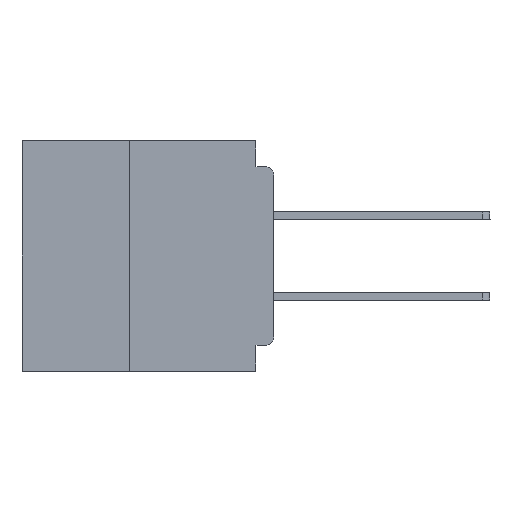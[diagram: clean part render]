
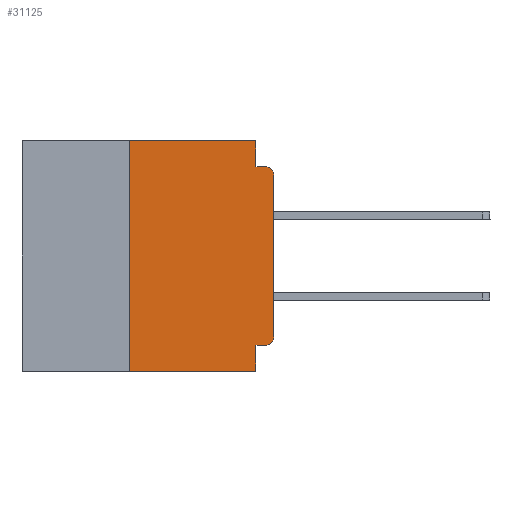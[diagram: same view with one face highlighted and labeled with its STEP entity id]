
A CAD part, left-side view. The second image highlights one B-rep face of the part: STEP entity #31125.
In plain terms, the highlighted planar face has unit normal (-1, 0, 0).
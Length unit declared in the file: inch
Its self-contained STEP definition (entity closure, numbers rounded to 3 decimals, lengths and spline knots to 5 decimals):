
#2431 = CARTESIAN_POINT ( 'NONE',  ( 0., 0.015, -0.34 ) ) ;
#4102 = PLANE ( 'NONE',  #14447 ) ;
#5259 = CARTESIAN_POINT ( 'NONE',  ( 0., 0.031, -0.045 ) ) ;
#5685 = CARTESIAN_POINT ( 'NONE',  ( 0., 0., -0.355 ) ) ;
#7285 = CARTESIAN_POINT ( 'NONE',  ( 0., 0., -0.045 ) ) ;
#7587 = DIRECTION ( 'NONE',  ( 0., 0., -1. ) ) ;
#7605 = ORIENTED_EDGE ( 'NONE', *, *, #59686, .F. ) ;
#8514 = VECTOR ( 'NONE', #66152, 39.37008 ) ;
#8557 = CARTESIAN_POINT ( 'NONE',  ( 0., 0., 0. ) ) ;
#10841 = AXIS2_PLACEMENT_3D ( 'NONE', #59793, #29209, #64865 ) ;
#10844 = DIRECTION ( 'NONE',  ( 0., 1., 0. ) ) ;
#11121 = VERTEX_POINT ( 'NONE', #42803 ) ;
#11649 = VECTOR ( 'NONE', #18840, 39.37008 ) ;
#12291 = AXIS2_PLACEMENT_3D ( 'NONE', #2431, #38357, #7587 ) ;
#12451 = DIRECTION ( 'NONE',  ( 0., -1., 0. ) ) ;
#13256 = VERTEX_POINT ( 'NONE', #27277 ) ;
#13714 = DIRECTION ( 'NONE',  ( 0., 0., 1. ) ) ;
#13742 = LINE ( 'NONE', #7285, #25807 ) ;
#14447 = AXIS2_PLACEMENT_3D ( 'NONE', #50246, #19533, #55405 ) ;
#15932 = ORIENTED_EDGE ( 'NONE', *, *, #49426, .T. ) ;
#17462 = VERTEX_POINT ( 'NONE', #36136 ) ;
#18364 = EDGE_CURVE ( 'NONE', #42436, #30151, #13742, .T. ) ;
#18504 = VECTOR ( 'NONE', #10844, 39.37008 ) ;
#18840 = DIRECTION ( 'NONE',  ( 0., 0., -1. ) ) ;
#18987 = VERTEX_POINT ( 'NONE', #60850 ) ;
#19533 = DIRECTION ( 'NONE',  ( 1., 0., 0. ) ) ;
#19624 = CARTESIAN_POINT ( 'NONE',  ( 0., 0.015, -0.355 ) ) ;
#20550 = EDGE_CURVE ( 'NONE', #44122, #23232, #44822, .T. ) ;
#21375 = CARTESIAN_POINT ( 'NONE',  ( 0., 0.031, -0.355 ) ) ;
#21750 = LINE ( 'NONE', #5685, #18504 ) ;
#23232 = VERTEX_POINT ( 'NONE', #45274 ) ;
#23278 = FACE_OUTER_BOUND ( 'NONE', #48159, .T. ) ;
#24277 = LINE ( 'NONE', #8557, #49921 ) ;
#24663 = CARTESIAN_POINT ( 'NONE',  ( 0., 0.437, -0.4 ) ) ;
#25420 = EDGE_CURVE ( 'NONE', #18987, #42436, #64444, .T. ) ;
#25807 = VECTOR ( 'NONE', #12451, 39.37008 ) ;
#27022 = ORIENTED_EDGE ( 'NONE', *, *, #25420, .F. ) ;
#27277 = CARTESIAN_POINT ( 'NONE',  ( 0., 0.25, -0.4 ) ) ;
#27496 = ORIENTED_EDGE ( 'NONE', *, *, #42465, .F. ) ;
#28491 = VECTOR ( 'NONE', #50415, 39.37008 ) ;
#28843 = LINE ( 'NONE', #61373, #42438 ) ;
#29209 = DIRECTION ( 'NONE',  ( -1., 0., 0. ) ) ;
#30151 = VERTEX_POINT ( 'NONE', #47084 ) ;
#30703 = CARTESIAN_POINT ( 'NONE',  ( 0., 0.437, 0. ) ) ;
#30791 = DIRECTION ( 'NONE',  ( 0., 0., 1. ) ) ;
#31125 = ADVANCED_FACE ( 'NONE', ( #23278 ), #4102, .F. ) ;
#33913 = VECTOR ( 'NONE', #36977, 39.37008 ) ;
#35733 = EDGE_CURVE ( 'NONE', #13256, #17462, #28843, .T. ) ;
#35987 = ORIENTED_EDGE ( 'NONE', *, *, #55439, .T. ) ;
#36136 = CARTESIAN_POINT ( 'NONE',  ( 0., 0.25, 0. ) ) ;
#36977 = DIRECTION ( 'NONE',  ( 0., 0., -1. ) ) ;
#38357 = DIRECTION ( 'NONE',  ( -1., 0., 0. ) ) ;
#38989 = CIRCLE ( 'NONE', #10841, 0.015 ) ;
#39714 = ORIENTED_EDGE ( 'NONE', *, *, #55824, .F. ) ;
#39793 = ORIENTED_EDGE ( 'NONE', *, *, #35733, .F. ) ;
#40507 = CARTESIAN_POINT ( 'NONE',  ( 0., 0., -0.06 ) ) ;
#42109 = LINE ( 'NONE', #24663, #28491 ) ;
#42371 = ORIENTED_EDGE ( 'NONE', *, *, #18364, .F. ) ;
#42436 = VERTEX_POINT ( 'NONE', #5259 ) ;
#42438 = VECTOR ( 'NONE', #30791, 39.37008 ) ;
#42465 = EDGE_CURVE ( 'NONE', #44122, #54715, #21750, .T. ) ;
#42803 = CARTESIAN_POINT ( 'NONE',  ( 0., 0.031, -0.4 ) ) ;
#44122 = VERTEX_POINT ( 'NONE', #19624 ) ;
#44822 = CIRCLE ( 'NONE', #12291, 0.015 ) ;
#45274 = CARTESIAN_POINT ( 'NONE',  ( 0., 0., -0.34 ) ) ;
#47043 = CARTESIAN_POINT ( 'NONE',  ( 0., 0.031, -0.4 ) ) ;
#47084 = CARTESIAN_POINT ( 'NONE',  ( 0., 0.015, -0.045 ) ) ;
#47502 = LINE ( 'NONE', #47043, #33913 ) ;
#48159 = EDGE_LOOP ( 'NONE', ( #65032, #35987, #42371, #27022, #39714, #39793, #15932, #7605, #27496, #49016 ) ) ;
#49016 = ORIENTED_EDGE ( 'NONE', *, *, #20550, .T. ) ;
#49426 = EDGE_CURVE ( 'NONE', #13256, #11121, #42109, .T. ) ;
#49921 = VECTOR ( 'NONE', #13714, 39.37008 ) ;
#50246 = CARTESIAN_POINT ( 'NONE',  ( 0., 0.437, 0. ) ) ;
#50415 = DIRECTION ( 'NONE',  ( 0., -1., 0. ) ) ;
#50600 = EDGE_CURVE ( 'NONE', #23232, #54544, #24277, .T. ) ;
#54544 = VERTEX_POINT ( 'NONE', #40507 ) ;
#54715 = VERTEX_POINT ( 'NONE', #21375 ) ;
#55405 = DIRECTION ( 'NONE',  ( 0., 0., -1. ) ) ;
#55439 = EDGE_CURVE ( 'NONE', #54544, #30151, #38989, .T. ) ;
#55824 = EDGE_CURVE ( 'NONE', #17462, #18987, #61394, .T. ) ;
#59686 = EDGE_CURVE ( 'NONE', #54715, #11121, #47502, .T. ) ;
#59793 = CARTESIAN_POINT ( 'NONE',  ( 0., 0.015, -0.06 ) ) ;
#59817 = CARTESIAN_POINT ( 'NONE',  ( 0., 0.031, 0. ) ) ;
#60850 = CARTESIAN_POINT ( 'NONE',  ( 0., 0.031, 0. ) ) ;
#61373 = CARTESIAN_POINT ( 'NONE',  ( 0., 0.25, -0.4 ) ) ;
#61394 = LINE ( 'NONE', #30703, #8514 ) ;
#64444 = LINE ( 'NONE', #59817, #11649 ) ;
#64865 = DIRECTION ( 'NONE',  ( 0., 0., -1. ) ) ;
#65032 = ORIENTED_EDGE ( 'NONE', *, *, #50600, .T. ) ;
#66152 = DIRECTION ( 'NONE',  ( 0., -1., 0. ) ) ;
